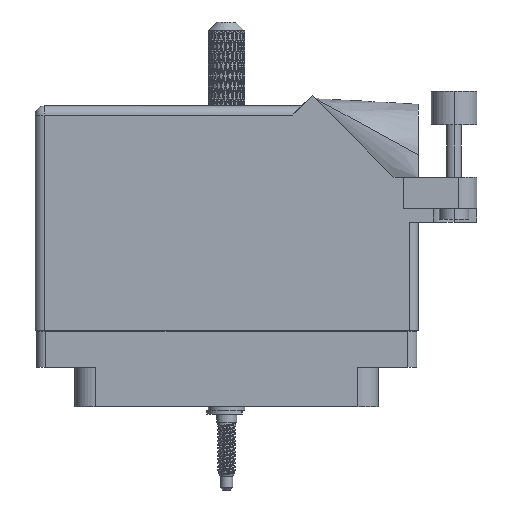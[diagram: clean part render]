
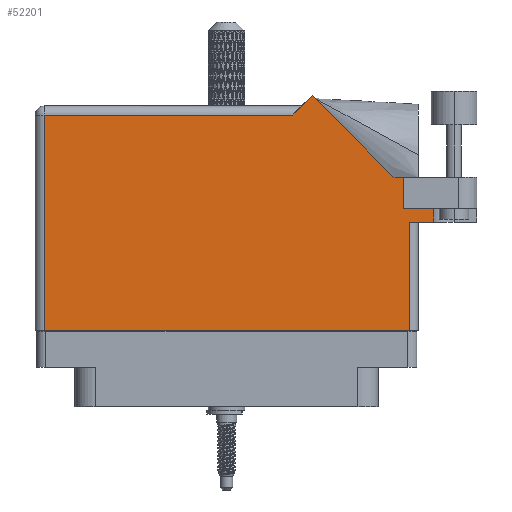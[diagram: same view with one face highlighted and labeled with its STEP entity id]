
A CAD part, front view. The second image highlights one B-rep face of the part: STEP entity #52201.
In plain terms, the highlighted face is planar.
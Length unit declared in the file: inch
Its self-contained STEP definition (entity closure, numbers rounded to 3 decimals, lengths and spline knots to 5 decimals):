
#1772 = ORIENTED_EDGE ( 'NONE', *, *, #92105, .T. ) ;
#2770 = AXIS2_PLACEMENT_3D ( 'NONE', #4248, #12993, #113306 ) ;
#4248 = CARTESIAN_POINT ( 'NONE',  ( -1.306, 1.43, 0.455 ) ) ;
#5485 = DIRECTION ( 'NONE',  ( 1., 0., 0. ) ) ;
#8895 = VERTEX_POINT ( 'NONE', #97449 ) ;
#9172 = LINE ( 'NONE', #92179, #37714 ) ;
#11603 = VERTEX_POINT ( 'NONE', #71758 ) ;
#11890 = CARTESIAN_POINT ( 'NONE',  ( 1.4075, 0.637, 0.455 ) ) ;
#12488 = ORIENTED_EDGE ( 'NONE', *, *, #105264, .T. ) ;
#12993 = DIRECTION ( 'NONE',  ( 0., 0., -1. ) ) ;
#13438 = LINE ( 'NONE', #112001, #83232 ) ;
#13695 = VECTOR ( 'NONE', #65620, 39.37008 ) ;
#16215 = LINE ( 'NONE', #105110, #110252 ) ;
#16895 = CARTESIAN_POINT ( 'NONE',  ( 1.244, 0.637, 0.455 ) ) ;
#17662 = DIRECTION ( 'NONE',  ( 0., -1., 0. ) ) ;
#18733 = LINE ( 'NONE', #16895, #117091 ) ;
#19396 = LINE ( 'NONE', #52908, #13695 ) ;
#20068 = DIRECTION ( 'NONE',  ( 1., 0., 0. ) ) ;
#20979 = ORIENTED_EDGE ( 'NONE', *, *, #44079, .T. ) ;
#22586 = CARTESIAN_POINT ( 'NONE',  ( 0.451, 1.368, 0.455 ) ) ;
#26406 = CARTESIAN_POINT ( 'NONE',  ( -1.244, -0.1, 0.455 ) ) ;
#27522 = VECTOR ( 'NONE', #66293, 39.37008 ) ;
#28952 = ORIENTED_EDGE ( 'NONE', *, *, #108064, .F. ) ;
#31360 = EDGE_CURVE ( 'NONE', #57054, #111834, #50696, .T. ) ;
#32549 = ORIENTED_EDGE ( 'NONE', *, *, #112950, .T. ) ;
#32787 = VECTOR ( 'NONE', #91035, 39.37008 ) ;
#33475 = DIRECTION ( 'NONE',  ( -1., 0., 0. ) ) ;
#36786 = CARTESIAN_POINT ( 'NONE',  ( 1.14042, 0.944, 0.455 ) ) ;
#37248 = CARTESIAN_POINT ( 'NONE',  ( 0.513, 1.43, 0.455 ) ) ;
#37714 = VECTOR ( 'NONE', #46754, 39.37008 ) ;
#37879 = CARTESIAN_POINT ( 'NONE',  ( 1.206, 0.731, 0.455 ) ) ;
#38442 = LINE ( 'NONE', #37879, #98365 ) ;
#43050 = CARTESIAN_POINT ( 'NONE',  ( 0.58371, 1.50071, 0.455 ) ) ;
#44079 = EDGE_CURVE ( 'NONE', #78068, #57054, #16215, .T. ) ;
#46536 = EDGE_CURVE ( 'NONE', #105170, #70443, #13438, .T. ) ;
#46754 = DIRECTION ( 'NONE',  ( 1., 0., 0. ) ) ;
#46994 = LINE ( 'NONE', #37248, #32787 ) ;
#47263 = EDGE_CURVE ( 'NONE', #58448, #57204, #91599, .T. ) ;
#48592 = VERTEX_POINT ( 'NONE', #116308 ) ;
#49262 = CARTESIAN_POINT ( 'NONE',  ( 1.244, 0.637, 0.455 ) ) ;
#50696 = LINE ( 'NONE', #78802, #80596 ) ;
#51167 = VECTOR ( 'NONE', #5485, 39.37008 ) ;
#52201 = ADVANCED_FACE ( 'NONE', ( #55262 ), #102617, .F. ) ;
#52908 = CARTESIAN_POINT ( 'NONE',  ( 1.4075, 1.06177, 0.455 ) ) ;
#55262 = FACE_OUTER_BOUND ( 'NONE', #107560, .T. ) ;
#57054 = VERTEX_POINT ( 'NONE', #36786 ) ;
#57204 = VERTEX_POINT ( 'NONE', #104003 ) ;
#58271 = VERTEX_POINT ( 'NONE', #91535 ) ;
#58448 = VERTEX_POINT ( 'NONE', #22586 ) ;
#60617 = EDGE_CURVE ( 'NONE', #11603, #58271, #9172, .T. ) ;
#63190 = ORIENTED_EDGE ( 'NONE', *, *, #69859, .T. ) ;
#65620 = DIRECTION ( 'NONE',  ( 0., -1., 0. ) ) ;
#66016 = CARTESIAN_POINT ( 'NONE',  ( -1.306, -0.1, 0.455 ) ) ;
#66293 = DIRECTION ( 'NONE',  ( -1., 0., 0. ) ) ;
#69859 = EDGE_CURVE ( 'NONE', #57204, #8895, #97382, .T. ) ;
#70443 = VERTEX_POINT ( 'NONE', #11890 ) ;
#71758 = CARTESIAN_POINT ( 'NONE',  ( 1.206, 0.731, 0.455 ) ) ;
#72384 = ORIENTED_EDGE ( 'NONE', *, *, #46536, .T. ) ;
#75678 = ORIENTED_EDGE ( 'NONE', *, *, #60617, .F. ) ;
#78068 = VERTEX_POINT ( 'NONE', #106967 ) ;
#78802 = CARTESIAN_POINT ( 'NONE',  ( 1.14042, 0.944, 0.455 ) ) ;
#80596 = VECTOR ( 'NONE', #87996, 39.37008 ) ;
#83232 = VECTOR ( 'NONE', #20068, 39.37008 ) ;
#83331 = EDGE_CURVE ( 'NONE', #111834, #58448, #46994, .T. ) ;
#84990 = CARTESIAN_POINT ( 'NONE',  ( -1.306, 1.368, 0.455 ) ) ;
#87996 = DIRECTION ( 'NONE',  ( -0.707, 0.707, 0. ) ) ;
#88597 = DIRECTION ( 'NONE',  ( 0., 1., 0. ) ) ;
#88764 = VECTOR ( 'NONE', #17662, 39.37008 ) ;
#91035 = DIRECTION ( 'NONE',  ( -0.707, -0.707, 0. ) ) ;
#91204 = ORIENTED_EDGE ( 'NONE', *, *, #83331, .T. ) ;
#91535 = CARTESIAN_POINT ( 'NONE',  ( 1.4075, 0.731, 0.455 ) ) ;
#91599 = LINE ( 'NONE', #84990, #27522 ) ;
#92105 = EDGE_CURVE ( 'NONE', #11603, #78068, #38442, .T. ) ;
#92179 = CARTESIAN_POINT ( 'NONE',  ( 1.206, 0.731, 0.455 ) ) ;
#97382 = LINE ( 'NONE', #26406, #88764 ) ;
#97449 = CARTESIAN_POINT ( 'NONE',  ( -1.244, -0.1, 0.455 ) ) ;
#98168 = LINE ( 'NONE', #66016, #51167 ) ;
#98365 = VECTOR ( 'NONE', #101606, 39.37008 ) ;
#98404 = ORIENTED_EDGE ( 'NONE', *, *, #47263, .T. ) ;
#101606 = DIRECTION ( 'NONE',  ( 0., 1., 0. ) ) ;
#102617 = PLANE ( 'NONE',  #2770 ) ;
#104003 = CARTESIAN_POINT ( 'NONE',  ( -1.244, 1.368, 0.455 ) ) ;
#105110 = CARTESIAN_POINT ( 'NONE',  ( 1.706, 0.944, 0.455 ) ) ;
#105170 = VERTEX_POINT ( 'NONE', #49262 ) ;
#105264 = EDGE_CURVE ( 'NONE', #8895, #48592, #98168, .T. ) ;
#106967 = CARTESIAN_POINT ( 'NONE',  ( 1.206, 0.944, 0.455 ) ) ;
#107560 = EDGE_LOOP ( 'NONE', ( #12488, #32549, #72384, #28952, #75678, #1772, #20979, #108067, #91204, #98404, #63190 ) ) ;
#108064 = EDGE_CURVE ( 'NONE', #58271, #70443, #19396, .T. ) ;
#108067 = ORIENTED_EDGE ( 'NONE', *, *, #31360, .T. ) ;
#110252 = VECTOR ( 'NONE', #33475, 39.37008 ) ;
#111834 = VERTEX_POINT ( 'NONE', #43050 ) ;
#112001 = CARTESIAN_POINT ( 'NONE',  ( 1.306, 0.637, 0.455 ) ) ;
#112950 = EDGE_CURVE ( 'NONE', #48592, #105170, #18733, .T. ) ;
#113306 = DIRECTION ( 'NONE',  ( -1., 0., 0. ) ) ;
#116308 = CARTESIAN_POINT ( 'NONE',  ( 1.244, -0.1, 0.455 ) ) ;
#117091 = VECTOR ( 'NONE', #88597, 39.37008 ) ;
